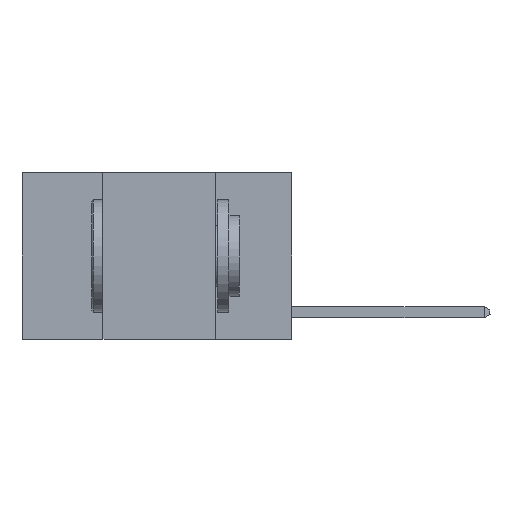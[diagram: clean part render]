
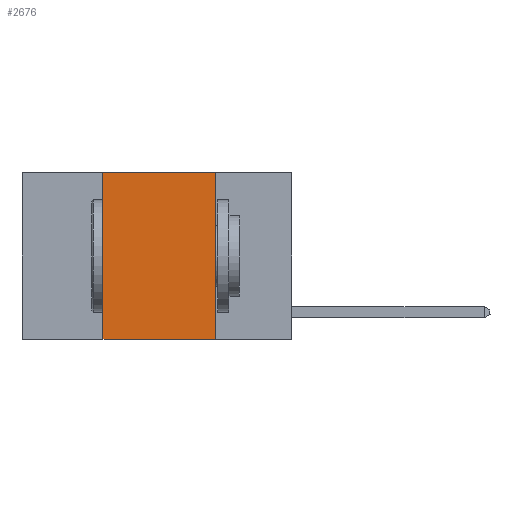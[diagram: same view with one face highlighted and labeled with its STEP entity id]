
A CAD part, left-side view. The second image highlights one B-rep face of the part: STEP entity #2676.
In plain terms, the highlighted planar face has unit normal (-1, 0, 0).
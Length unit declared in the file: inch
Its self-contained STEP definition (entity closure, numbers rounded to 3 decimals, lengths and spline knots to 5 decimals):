
#8 = CARTESIAN_POINT ( 'NONE',  ( 0., 0.6, 0. ) ) ;
#95 = EDGE_CURVE ( 'NONE', #5767, #4220, #12233, .T. ) ;
#527 = VECTOR ( 'NONE', #10801, 39.37008 ) ;
#934 = DIRECTION ( 'NONE',  ( 0., 0., -1. ) ) ;
#1535 = EDGE_CURVE ( 'NONE', #5767, #10221, #1828, .T. ) ;
#1554 = ORIENTED_EDGE ( 'NONE', *, *, #95, .T. ) ;
#1828 = LINE ( 'NONE', #6204, #527 ) ;
#2399 = CARTESIAN_POINT ( 'NONE',  ( 0., 0.6, -0.37 ) ) ;
#2460 = ORIENTED_EDGE ( 'NONE', *, *, #4295, .F. ) ;
#2676 = ADVANCED_FACE ( 'NONE', ( #10753 ), #9808, .F. ) ;
#3256 = AXIS2_PLACEMENT_3D ( 'NONE', #8, #5382, #934 ) ;
#3473 = VERTEX_POINT ( 'NONE', #14157 ) ;
#3870 = CARTESIAN_POINT ( 'NONE',  ( 0., 0.42, 0. ) ) ;
#4220 = VERTEX_POINT ( 'NONE', #13757 ) ;
#4295 = EDGE_CURVE ( 'NONE', #3473, #4220, #12884, .T. ) ;
#5382 = DIRECTION ( 'NONE',  ( 1., 0., 0. ) ) ;
#5767 = VERTEX_POINT ( 'NONE', #9495 ) ;
#5907 = ORIENTED_EDGE ( 'NONE', *, *, #1535, .F. ) ;
#6204 = CARTESIAN_POINT ( 'NONE',  ( 0., 0.42, 0. ) ) ;
#6487 = VECTOR ( 'NONE', #13096, 39.37008 ) ;
#6779 = DIRECTION ( 'NONE',  ( 0., -1., 0. ) ) ;
#7306 = VECTOR ( 'NONE', #6779, 39.37008 ) ;
#7418 = CARTESIAN_POINT ( 'NONE',  ( 0., 0.17, 0. ) ) ;
#8198 = DIRECTION ( 'NONE',  ( 0., -1., 0. ) ) ;
#9148 = LINE ( 'NONE', #9367, #12807 ) ;
#9367 = CARTESIAN_POINT ( 'NONE',  ( 0., 0.6, 0. ) ) ;
#9495 = CARTESIAN_POINT ( 'NONE',  ( 0., 0.42, -0.37 ) ) ;
#9756 = ORIENTED_EDGE ( 'NONE', *, *, #13327, .F. ) ;
#9808 = PLANE ( 'NONE',  #3256 ) ;
#10221 = VERTEX_POINT ( 'NONE', #3870 ) ;
#10753 = FACE_OUTER_BOUND ( 'NONE', #12601, .T. ) ;
#10801 = DIRECTION ( 'NONE',  ( 0., 0., 1. ) ) ;
#12233 = LINE ( 'NONE', #2399, #7306 ) ;
#12601 = EDGE_LOOP ( 'NONE', ( #2460, #9756, #5907, #1554 ) ) ;
#12807 = VECTOR ( 'NONE', #8198, 39.37008 ) ;
#12884 = LINE ( 'NONE', #7418, #6487 ) ;
#13096 = DIRECTION ( 'NONE',  ( 0., 0., -1. ) ) ;
#13327 = EDGE_CURVE ( 'NONE', #10221, #3473, #9148, .T. ) ;
#13757 = CARTESIAN_POINT ( 'NONE',  ( 0., 0.17, -0.37 ) ) ;
#14157 = CARTESIAN_POINT ( 'NONE',  ( 0., 0.17, 0. ) ) ;
